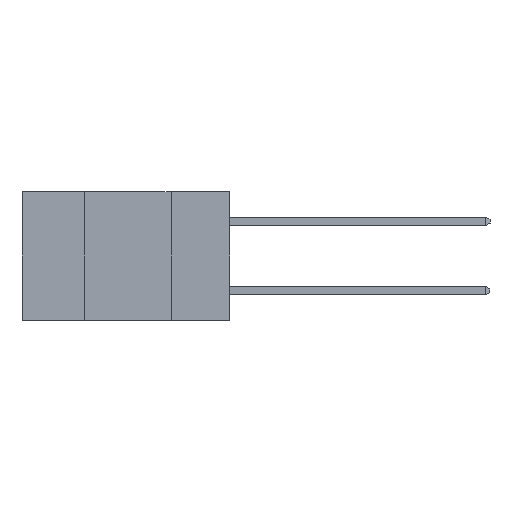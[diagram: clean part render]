
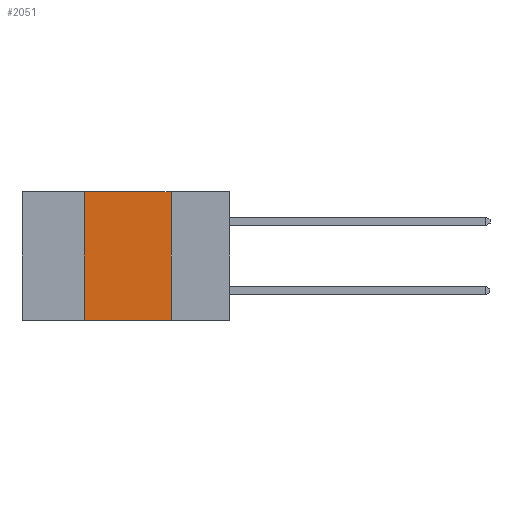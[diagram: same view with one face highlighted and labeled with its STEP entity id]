
A CAD part, left-side view. The second image highlights one B-rep face of the part: STEP entity #2051.
In plain terms, the highlighted planar face has unit normal (-1, 0, 0).
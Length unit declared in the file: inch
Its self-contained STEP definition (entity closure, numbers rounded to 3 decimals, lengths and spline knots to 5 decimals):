
#269 = CARTESIAN_POINT ( 'NONE',  ( 0., 0.6, -0.37 ) ) ;
#404 = EDGE_CURVE ( 'NONE', #14174, #8741, #4789, .T. ) ;
#1536 = EDGE_CURVE ( 'NONE', #8741, #7149, #12946, .T. ) ;
#1678 = EDGE_CURVE ( 'NONE', #7149, #6013, #8738, .T. ) ;
#2051 = ADVANCED_FACE ( 'NONE', ( #9304 ), #3808, .F. ) ;
#2189 = VECTOR ( 'NONE', #12417, 39.37008 ) ;
#3342 = DIRECTION ( 'NONE',  ( 1., 0., 0. ) ) ;
#3808 = PLANE ( 'NONE',  #4043 ) ;
#4043 = AXIS2_PLACEMENT_3D ( 'NONE', #4062, #3342, #4115 ) ;
#4062 = CARTESIAN_POINT ( 'NONE',  ( 0., 0.6, 0. ) ) ;
#4115 = DIRECTION ( 'NONE',  ( 0., 0., -1. ) ) ;
#4167 = VECTOR ( 'NONE', #10039, 39.37008 ) ;
#4293 = VECTOR ( 'NONE', #19160, 39.37008 ) ;
#4589 = CARTESIAN_POINT ( 'NONE',  ( 0., 0.42, 0. ) ) ;
#4789 = LINE ( 'NONE', #20343, #4167 ) ;
#5982 = CARTESIAN_POINT ( 'NONE',  ( 0., 0.42, -0.37 ) ) ;
#6013 = VERTEX_POINT ( 'NONE', #21121 ) ;
#7149 = VERTEX_POINT ( 'NONE', #22845 ) ;
#7598 = LINE ( 'NONE', #269, #21814 ) ;
#8490 = ORIENTED_EDGE ( 'NONE', *, *, #24087, .T. ) ;
#8738 = LINE ( 'NONE', #19243, #4293 ) ;
#8741 = VERTEX_POINT ( 'NONE', #4589 ) ;
#9304 = FACE_OUTER_BOUND ( 'NONE', #10918, .T. ) ;
#10039 = DIRECTION ( 'NONE',  ( 0., 0., 1. ) ) ;
#10083 = CARTESIAN_POINT ( 'NONE',  ( 0., 0.6, 0. ) ) ;
#10918 = EDGE_LOOP ( 'NONE', ( #12363, #22730, #18179, #8490 ) ) ;
#12363 = ORIENTED_EDGE ( 'NONE', *, *, #1678, .F. ) ;
#12417 = DIRECTION ( 'NONE',  ( 0., -1., 0. ) ) ;
#12946 = LINE ( 'NONE', #10083, #2189 ) ;
#14174 = VERTEX_POINT ( 'NONE', #5982 ) ;
#18179 = ORIENTED_EDGE ( 'NONE', *, *, #404, .F. ) ;
#19160 = DIRECTION ( 'NONE',  ( 0., 0., -1. ) ) ;
#19243 = CARTESIAN_POINT ( 'NONE',  ( 0., 0.17, 0. ) ) ;
#20343 = CARTESIAN_POINT ( 'NONE',  ( 0., 0.42, 0. ) ) ;
#21121 = CARTESIAN_POINT ( 'NONE',  ( 0., 0.17, -0.37 ) ) ;
#21589 = DIRECTION ( 'NONE',  ( 0., -1., 0. ) ) ;
#21814 = VECTOR ( 'NONE', #21589, 39.37008 ) ;
#22730 = ORIENTED_EDGE ( 'NONE', *, *, #1536, .F. ) ;
#22845 = CARTESIAN_POINT ( 'NONE',  ( 0., 0.17, 0. ) ) ;
#24087 = EDGE_CURVE ( 'NONE', #14174, #6013, #7598, .T. ) ;
